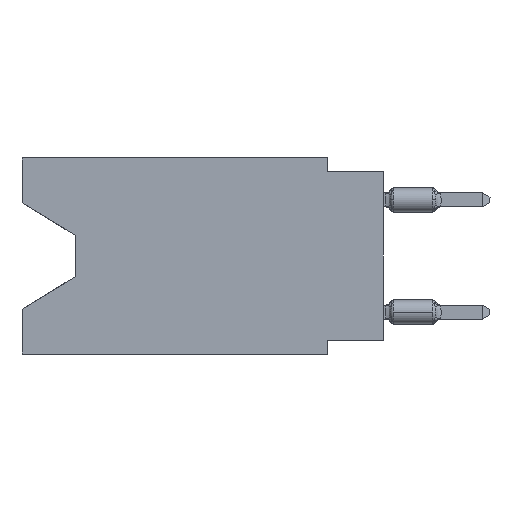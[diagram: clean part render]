
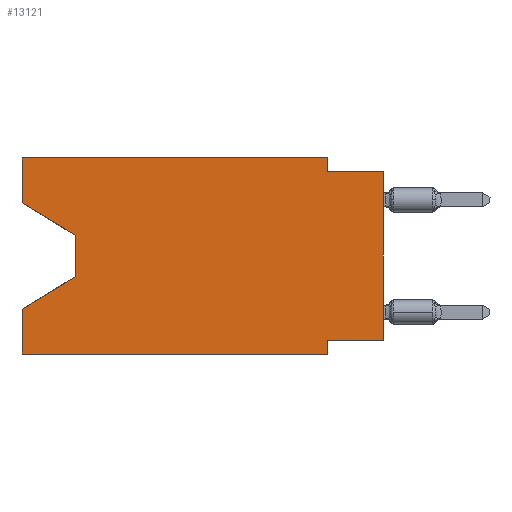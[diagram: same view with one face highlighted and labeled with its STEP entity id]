
A CAD part, left-side view. The second image highlights one B-rep face of the part: STEP entity #13121.
In plain terms, the highlighted planar face has unit normal (-1, 0, 0).
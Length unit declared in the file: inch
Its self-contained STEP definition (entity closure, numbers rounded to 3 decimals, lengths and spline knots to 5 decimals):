
#364 = DIRECTION ( 'NONE',  ( 0., -1., 0. ) ) ;
#778 = CARTESIAN_POINT ( 'NONE',  ( 0., 0.1, -0.325 ) ) ;
#875 = CARTESIAN_POINT ( 'NONE',  ( 0., 0.1, 0. ) ) ;
#1322 = EDGE_CURVE ( 'NONE', #6514, #27775, #15367, .T. ) ;
#1447 = DIRECTION ( 'NONE',  ( 0., -0.855, -0.519 ) ) ;
#1576 = VECTOR ( 'NONE', #9210, 39.37008 ) ;
#1952 = DIRECTION ( 'NONE',  ( 0., 0., -1. ) ) ;
#2262 = LINE ( 'NONE', #11447, #17363 ) ;
#2709 = VERTEX_POINT ( 'NONE', #8977 ) ;
#2810 = CARTESIAN_POINT ( 'NONE',  ( 0., 0., -0.025 ) ) ;
#3926 = ORIENTED_EDGE ( 'NONE', *, *, #24856, .F. ) ;
#4095 = ORIENTED_EDGE ( 'NONE', *, *, #27151, .T. ) ;
#4273 = LINE ( 'NONE', #28572, #26642 ) ;
#4359 = EDGE_CURVE ( 'NONE', #19827, #12280, #2262, .T. ) ;
#4373 = ORIENTED_EDGE ( 'NONE', *, *, #15474, .F. ) ;
#5224 = CARTESIAN_POINT ( 'NONE',  ( 0., 0.645, -0.26975 ) ) ;
#5663 = CARTESIAN_POINT ( 'NONE',  ( 0., 0.55, -0.212 ) ) ;
#5839 = DIRECTION ( 'NONE',  ( 0., 1., 0. ) ) ;
#5867 = DIRECTION ( 'NONE',  ( 0., 0., 1. ) ) ;
#6029 = PLANE ( 'NONE',  #18687 ) ;
#6514 = VERTEX_POINT ( 'NONE', #24576 ) ;
#7353 = DIRECTION ( 'NONE',  ( 0., 0.855, -0.519 ) ) ;
#7739 = VERTEX_POINT ( 'NONE', #21565 ) ;
#7926 = LINE ( 'NONE', #26294, #15874 ) ;
#7955 = LINE ( 'NONE', #26322, #19551 ) ;
#8977 = CARTESIAN_POINT ( 'NONE',  ( 0., 0.1, 0. ) ) ;
#9210 = DIRECTION ( 'NONE',  ( 0., 0., 1. ) ) ;
#9360 = DIRECTION ( 'NONE',  ( 0., 0., -1. ) ) ;
#9917 = VERTEX_POINT ( 'NONE', #15833 ) ;
#10153 = VECTOR ( 'NONE', #364, 39.37008 ) ;
#10581 = VECTOR ( 'NONE', #11852, 39.37008 ) ;
#10845 = EDGE_CURVE ( 'NONE', #9917, #14152, #7955, .T. ) ;
#10881 = EDGE_CURVE ( 'NONE', #9917, #12280, #12698, .T. ) ;
#10889 = CARTESIAN_POINT ( 'NONE',  ( 0., 0.645, -0.08025 ) ) ;
#11124 = CARTESIAN_POINT ( 'NONE',  ( 0., 0.55, -0.138 ) ) ;
#11447 = CARTESIAN_POINT ( 'NONE',  ( 0., 0.1, -0.35 ) ) ;
#11644 = VECTOR ( 'NONE', #13209, 39.37008 ) ;
#11718 = LINE ( 'NONE', #14233, #1576 ) ;
#11852 = DIRECTION ( 'NONE',  ( 0., -1., 0. ) ) ;
#12280 = VERTEX_POINT ( 'NONE', #19181 ) ;
#12698 = LINE ( 'NONE', #15324, #18132 ) ;
#13121 = ADVANCED_FACE ( 'NONE', ( #17273 ), #6029, .F. ) ;
#13209 = DIRECTION ( 'NONE',  ( 0., 0., -1. ) ) ;
#13643 = ORIENTED_EDGE ( 'NONE', *, *, #28094, .F. ) ;
#14098 = LINE ( 'NONE', #2810, #10581 ) ;
#14152 = VERTEX_POINT ( 'NONE', #5224 ) ;
#14227 = VERTEX_POINT ( 'NONE', #5663 ) ;
#14233 = CARTESIAN_POINT ( 'NONE',  ( 0., 0.645, 0. ) ) ;
#14880 = ORIENTED_EDGE ( 'NONE', *, *, #28015, .F. ) ;
#15031 = VECTOR ( 'NONE', #26635, 39.37008 ) ;
#15056 = DIRECTION ( 'NONE',  ( 0., 0., -1. ) ) ;
#15324 = CARTESIAN_POINT ( 'NONE',  ( 0., 0.645, -0.35 ) ) ;
#15367 = LINE ( 'NONE', #17436, #15031 ) ;
#15474 = EDGE_CURVE ( 'NONE', #6514, #19827, #7926, .T. ) ;
#15833 = CARTESIAN_POINT ( 'NONE',  ( 0., 0.645, -0.35 ) ) ;
#15842 = ORIENTED_EDGE ( 'NONE', *, *, #10881, .T. ) ;
#15874 = VECTOR ( 'NONE', #5839, 39.37008 ) ;
#16641 = VECTOR ( 'NONE', #9360, 39.37008 ) ;
#17114 = CARTESIAN_POINT ( 'NONE',  ( 0., 0.645, 0. ) ) ;
#17273 = FACE_OUTER_BOUND ( 'NONE', #17643, .T. ) ;
#17363 = VECTOR ( 'NONE', #1952, 39.37008 ) ;
#17436 = CARTESIAN_POINT ( 'NONE',  ( 0., 0., 0. ) ) ;
#17451 = VERTEX_POINT ( 'NONE', #25197 ) ;
#17643 = EDGE_LOOP ( 'NONE', ( #4095, #27862, #22176, #19750, #15842, #19034, #4373, #24902, #13643, #3926, #29261, #14880 ) ) ;
#18132 = VECTOR ( 'NONE', #28246, 39.37008 ) ;
#18687 = AXIS2_PLACEMENT_3D ( 'NONE', #17114, #19926, #15056 ) ;
#18894 = CARTESIAN_POINT ( 'NONE',  ( 0., 0.55, -0.212 ) ) ;
#19034 = ORIENTED_EDGE ( 'NONE', *, *, #4359, .F. ) ;
#19181 = CARTESIAN_POINT ( 'NONE',  ( 0., 0.1, -0.35 ) ) ;
#19551 = VECTOR ( 'NONE', #5867, 39.37008 ) ;
#19750 = ORIENTED_EDGE ( 'NONE', *, *, #10845, .F. ) ;
#19827 = VERTEX_POINT ( 'NONE', #778 ) ;
#19866 = LINE ( 'NONE', #11124, #11644 ) ;
#19926 = DIRECTION ( 'NONE',  ( 1., 0., 0. ) ) ;
#21411 = LINE ( 'NONE', #18894, #25792 ) ;
#21565 = CARTESIAN_POINT ( 'NONE',  ( 0., 0.55, -0.138 ) ) ;
#21664 = CARTESIAN_POINT ( 'NONE',  ( 0., 0., -0.025 ) ) ;
#22176 = ORIENTED_EDGE ( 'NONE', *, *, #29081, .T. ) ;
#22579 = CARTESIAN_POINT ( 'NONE',  ( 0., 0.1, -0.025 ) ) ;
#22615 = VERTEX_POINT ( 'NONE', #10889 ) ;
#23067 = CARTESIAN_POINT ( 'NONE',  ( 0., 0.645, 0. ) ) ;
#23434 = LINE ( 'NONE', #875, #16641 ) ;
#23454 = EDGE_CURVE ( 'NONE', #7739, #14227, #19866, .T. ) ;
#24576 = CARTESIAN_POINT ( 'NONE',  ( 0., 0., -0.325 ) ) ;
#24856 = EDGE_CURVE ( 'NONE', #2709, #29308, #23434, .T. ) ;
#24902 = ORIENTED_EDGE ( 'NONE', *, *, #1322, .T. ) ;
#24994 = LINE ( 'NONE', #23067, #10153 ) ;
#25197 = CARTESIAN_POINT ( 'NONE',  ( 0., 0.645, 0. ) ) ;
#25792 = VECTOR ( 'NONE', #7353, 39.37008 ) ;
#26294 = CARTESIAN_POINT ( 'NONE',  ( 0., 0., -0.325 ) ) ;
#26322 = CARTESIAN_POINT ( 'NONE',  ( 0., 0.645, 0. ) ) ;
#26635 = DIRECTION ( 'NONE',  ( 0., 0., 1. ) ) ;
#26642 = VECTOR ( 'NONE', #1447, 39.37008 ) ;
#27151 = EDGE_CURVE ( 'NONE', #22615, #7739, #4273, .T. ) ;
#27775 = VERTEX_POINT ( 'NONE', #21664 ) ;
#27862 = ORIENTED_EDGE ( 'NONE', *, *, #23454, .T. ) ;
#28015 = EDGE_CURVE ( 'NONE', #22615, #17451, #11718, .T. ) ;
#28094 = EDGE_CURVE ( 'NONE', #29308, #27775, #14098, .T. ) ;
#28246 = DIRECTION ( 'NONE',  ( 0., -1., 0. ) ) ;
#28572 = CARTESIAN_POINT ( 'NONE',  ( 0., 0.645, -0.08025 ) ) ;
#28876 = EDGE_CURVE ( 'NONE', #17451, #2709, #24994, .T. ) ;
#29081 = EDGE_CURVE ( 'NONE', #14227, #14152, #21411, .T. ) ;
#29261 = ORIENTED_EDGE ( 'NONE', *, *, #28876, .F. ) ;
#29308 = VERTEX_POINT ( 'NONE', #22579 ) ;
